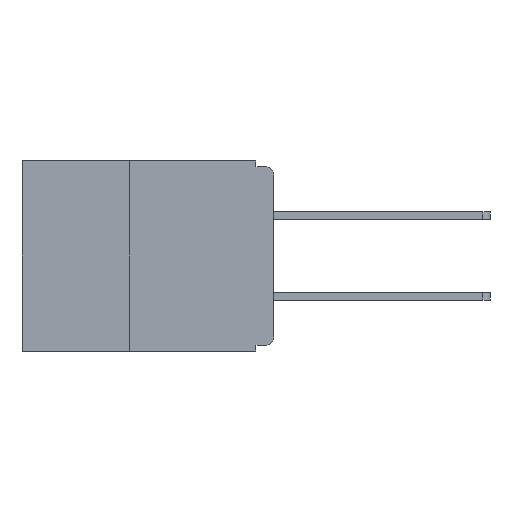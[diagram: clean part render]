
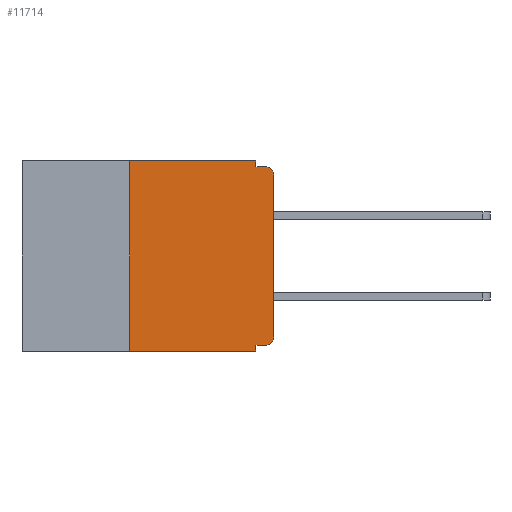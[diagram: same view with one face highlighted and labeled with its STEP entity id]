
A CAD part, left-side view. The second image highlights one B-rep face of the part: STEP entity #11714.
In plain terms, the highlighted planar face has unit normal (-1, 0, 0).
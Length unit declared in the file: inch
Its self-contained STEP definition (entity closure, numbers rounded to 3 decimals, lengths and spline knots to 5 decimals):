
#2 = VERTEX_POINT ( 'NONE', #10182 ) ;
#311 = EDGE_CURVE ( 'NONE', #9332, #9594, #4783, .T. ) ;
#633 = VECTOR ( 'NONE', #1927, 39.37008 ) ;
#637 = LINE ( 'NONE', #2307, #633 ) ;
#659 = EDGE_CURVE ( 'NONE', #2, #7031, #2487, .T. ) ;
#1155 = CARTESIAN_POINT ( 'NONE',  ( 0., 0.031, -0.32 ) ) ;
#1701 = DIRECTION ( 'NONE',  ( 0., 0., -1. ) ) ;
#1927 = DIRECTION ( 'NONE',  ( 0., 0., -1. ) ) ;
#1966 = DIRECTION ( 'NONE',  ( 1., 0., 0. ) ) ;
#2307 = CARTESIAN_POINT ( 'NONE',  ( 0., 0.031, -0.33 ) ) ;
#2449 = PLANE ( 'NONE',  #10054 ) ;
#2487 = LINE ( 'NONE', #8899, #2558 ) ;
#2558 = VECTOR ( 'NONE', #6366, 39.37008 ) ;
#2976 = VERTEX_POINT ( 'NONE', #5720 ) ;
#3284 = CARTESIAN_POINT ( 'NONE',  ( 0., 0.437, 0. ) ) ;
#3615 = CARTESIAN_POINT ( 'NONE',  ( 0., 0.25, -0.33 ) ) ;
#3678 = CARTESIAN_POINT ( 'NONE',  ( 0., 0., -0.305 ) ) ;
#3901 = EDGE_CURVE ( 'NONE', #12860, #9594, #7359, .T. ) ;
#4063 = ORIENTED_EDGE ( 'NONE', *, *, #9119, .T. ) ;
#4192 = FACE_OUTER_BOUND ( 'NONE', #8951, .T. ) ;
#4579 = ORIENTED_EDGE ( 'NONE', *, *, #311, .T. ) ;
#4735 = VECTOR ( 'NONE', #7621, 39.37008 ) ;
#4783 = CIRCLE ( 'NONE', #12595, 0.015 ) ;
#5068 = CARTESIAN_POINT ( 'NONE',  ( 0., 0.031, -0.01 ) ) ;
#5124 = CARTESIAN_POINT ( 'NONE',  ( 0., 0., -0.025 ) ) ;
#5134 = CARTESIAN_POINT ( 'NONE',  ( 0., 0.25, 0. ) ) ;
#5483 = EDGE_CURVE ( 'NONE', #6511, #2976, #5812, .T. ) ;
#5556 = CARTESIAN_POINT ( 'NONE',  ( 0., 0.031, 0. ) ) ;
#5593 = EDGE_CURVE ( 'NONE', #7910, #11637, #11116, .T. ) ;
#5720 = CARTESIAN_POINT ( 'NONE',  ( 0., 0.031, -0.33 ) ) ;
#5812 = LINE ( 'NONE', #7662, #4735 ) ;
#5826 = CARTESIAN_POINT ( 'NONE',  ( 0., 0.437, 0. ) ) ;
#5860 = DIRECTION ( 'NONE',  ( 0., -1., 0. ) ) ;
#5893 = AXIS2_PLACEMENT_3D ( 'NONE', #6985, #6317, #7555 ) ;
#6071 = ORIENTED_EDGE ( 'NONE', *, *, #8792, .F. ) ;
#6187 = ORIENTED_EDGE ( 'NONE', *, *, #5593, .F. ) ;
#6276 = ORIENTED_EDGE ( 'NONE', *, *, #10922, .F. ) ;
#6317 = DIRECTION ( 'NONE',  ( -1., 0., 0. ) ) ;
#6343 = ORIENTED_EDGE ( 'NONE', *, *, #5483, .T. ) ;
#6366 = DIRECTION ( 'NONE',  ( 0., 1., 0. ) ) ;
#6452 = ORIENTED_EDGE ( 'NONE', *, *, #8130, .F. ) ;
#6504 = VERTEX_POINT ( 'NONE', #3678 ) ;
#6511 = VERTEX_POINT ( 'NONE', #3615 ) ;
#6555 = VECTOR ( 'NONE', #8510, 39.37008 ) ;
#6565 = LINE ( 'NONE', #8413, #6555 ) ;
#6600 = ORIENTED_EDGE ( 'NONE', *, *, #659, .F. ) ;
#6734 = ORIENTED_EDGE ( 'NONE', *, *, #8460, .T. ) ;
#6985 = CARTESIAN_POINT ( 'NONE',  ( 0., 0.015, -0.305 ) ) ;
#7031 = VERTEX_POINT ( 'NONE', #1155 ) ;
#7047 = ORIENTED_EDGE ( 'NONE', *, *, #3901, .F. ) ;
#7243 = VECTOR ( 'NONE', #9003, 39.37008 ) ;
#7359 = LINE ( 'NONE', #9759, #7243 ) ;
#7555 = DIRECTION ( 'NONE',  ( 0., 0., -1. ) ) ;
#7621 = DIRECTION ( 'NONE',  ( 0., -1., 0. ) ) ;
#7662 = CARTESIAN_POINT ( 'NONE',  ( 0., 0.437, -0.33 ) ) ;
#7910 = VERTEX_POINT ( 'NONE', #5134 ) ;
#8104 = DIRECTION ( 'NONE',  ( 0., 0., 1. ) ) ;
#8130 = EDGE_CURVE ( 'NONE', #7031, #2976, #637, .T. ) ;
#8413 = CARTESIAN_POINT ( 'NONE',  ( 0., 0.25, -0.33 ) ) ;
#8422 = CARTESIAN_POINT ( 'NONE',  ( 0., 0., 0. ) ) ;
#8460 = EDGE_CURVE ( 'NONE', #2, #6504, #12987, .T. ) ;
#8510 = DIRECTION ( 'NONE',  ( 0., 0., 1. ) ) ;
#8792 = EDGE_CURVE ( 'NONE', #11637, #12860, #12007, .T. ) ;
#8899 = CARTESIAN_POINT ( 'NONE',  ( 0., 0., -0.32 ) ) ;
#8951 = EDGE_LOOP ( 'NONE', ( #4063, #4579, #7047, #6071, #6187, #6276, #6343, #6452, #6600, #6734 ) ) ;
#9003 = DIRECTION ( 'NONE',  ( 0., -1., 0. ) ) ;
#9119 = EDGE_CURVE ( 'NONE', #6504, #9332, #11036, .T. ) ;
#9332 = VERTEX_POINT ( 'NONE', #5124 ) ;
#9594 = VERTEX_POINT ( 'NONE', #13252 ) ;
#9759 = CARTESIAN_POINT ( 'NONE',  ( 0., 0., -0.01 ) ) ;
#10011 = VECTOR ( 'NONE', #5860, 39.37008 ) ;
#10054 = AXIS2_PLACEMENT_3D ( 'NONE', #3284, #1966, #1701 ) ;
#10182 = CARTESIAN_POINT ( 'NONE',  ( 0., 0.015, -0.32 ) ) ;
#10895 = VECTOR ( 'NONE', #8104, 39.37008 ) ;
#10922 = EDGE_CURVE ( 'NONE', #6511, #7910, #6565, .T. ) ;
#11036 = LINE ( 'NONE', #8422, #10895 ) ;
#11116 = LINE ( 'NONE', #5826, #10011 ) ;
#11637 = VERTEX_POINT ( 'NONE', #5556 ) ;
#11714 = ADVANCED_FACE ( 'NONE', ( #4192 ), #2449, .F. ) ;
#11978 = VECTOR ( 'NONE', #12728, 39.37008 ) ;
#12007 = LINE ( 'NONE', #12805, #11978 ) ;
#12104 = CARTESIAN_POINT ( 'NONE',  ( 0., 0.015, -0.025 ) ) ;
#12127 = DIRECTION ( 'NONE',  ( 0., 0., -1. ) ) ;
#12195 = DIRECTION ( 'NONE',  ( -1., 0., 0. ) ) ;
#12595 = AXIS2_PLACEMENT_3D ( 'NONE', #12104, #12195, #12127 ) ;
#12728 = DIRECTION ( 'NONE',  ( 0., 0., -1. ) ) ;
#12805 = CARTESIAN_POINT ( 'NONE',  ( 0., 0.031, 0. ) ) ;
#12860 = VERTEX_POINT ( 'NONE', #5068 ) ;
#12987 = CIRCLE ( 'NONE', #5893, 0.015 ) ;
#13252 = CARTESIAN_POINT ( 'NONE',  ( 0., 0.015, -0.01 ) ) ;
